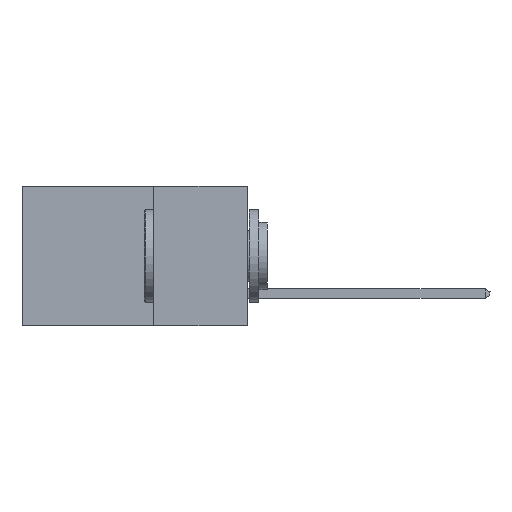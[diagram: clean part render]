
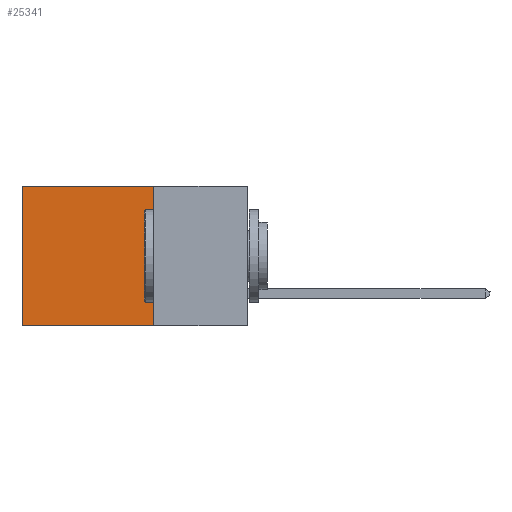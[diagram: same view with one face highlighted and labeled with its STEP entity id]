
A CAD part, left-side view. The second image highlights one B-rep face of the part: STEP entity #25341.
In plain terms, the highlighted planar face has unit normal (-1, 0, 0).
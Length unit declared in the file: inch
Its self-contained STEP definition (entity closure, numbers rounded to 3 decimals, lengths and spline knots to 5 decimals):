
#569 = LINE ( 'NONE', #8691, #19770 ) ;
#989 = EDGE_CURVE ( 'NONE', #20476, #14069, #7910, .T. ) ;
#1422 = VECTOR ( 'NONE', #15176, 39.37008 ) ;
#1435 = LINE ( 'NONE', #11559, #1422 ) ;
#1596 = AXIS2_PLACEMENT_3D ( 'NONE', #25720, #3160, #19194 ) ;
#2236 = VECTOR ( 'NONE', #13458, 39.37008 ) ;
#3160 = DIRECTION ( 'NONE',  ( 1., 0., 0. ) ) ;
#4863 = EDGE_CURVE ( 'NONE', #21299, #14069, #7465, .T. ) ;
#5056 = VERTEX_POINT ( 'NONE', #12913 ) ;
#5290 = PLANE ( 'NONE',  #1596 ) ;
#7465 = LINE ( 'NONE', #25747, #2236 ) ;
#7910 = LINE ( 'NONE', #13906, #25035 ) ;
#8293 = ORIENTED_EDGE ( 'NONE', *, *, #4863, .F. ) ;
#8383 = CARTESIAN_POINT ( 'NONE',  ( 0.2615, 0.6, -0.37 ) ) ;
#8691 = CARTESIAN_POINT ( 'NONE',  ( 0.2615, 0.25, -0.37 ) ) ;
#11559 = CARTESIAN_POINT ( 'NONE',  ( 0.2615, 0.25, 0. ) ) ;
#12913 = CARTESIAN_POINT ( 'NONE',  ( 0.2615, 0.25, 0. ) ) ;
#13458 = DIRECTION ( 'NONE',  ( 0., 1., 0. ) ) ;
#13906 = CARTESIAN_POINT ( 'NONE',  ( 0.2615, 0.6, -0.37 ) ) ;
#14069 = VERTEX_POINT ( 'NONE', #8383 ) ;
#15176 = DIRECTION ( 'NONE',  ( 0., 1., 0. ) ) ;
#16132 = CARTESIAN_POINT ( 'NONE',  ( 0.2615, 0.6, 0. ) ) ;
#16305 = CARTESIAN_POINT ( 'NONE',  ( 0.2615, 0.25, -0.37 ) ) ;
#17110 = DIRECTION ( 'NONE',  ( 0., 0., -1. ) ) ;
#17390 = ORIENTED_EDGE ( 'NONE', *, *, #989, .T. ) ;
#19194 = DIRECTION ( 'NONE',  ( 0., 0., -1. ) ) ;
#19270 = ORIENTED_EDGE ( 'NONE', *, *, #20813, .T. ) ;
#19770 = VECTOR ( 'NONE', #17110, 39.37008 ) ;
#20476 = VERTEX_POINT ( 'NONE', #16132 ) ;
#20813 = EDGE_CURVE ( 'NONE', #5056, #20476, #1435, .T. ) ;
#21299 = VERTEX_POINT ( 'NONE', #16305 ) ;
#21495 = EDGE_CURVE ( 'NONE', #5056, #21299, #569, .T. ) ;
#21979 = ORIENTED_EDGE ( 'NONE', *, *, #21495, .F. ) ;
#23473 = FACE_OUTER_BOUND ( 'NONE', #25352, .T. ) ;
#25035 = VECTOR ( 'NONE', #26339, 39.37008 ) ;
#25341 = ADVANCED_FACE ( 'NONE', ( #23473 ), #5290, .F. ) ;
#25352 = EDGE_LOOP ( 'NONE', ( #17390, #8293, #21979, #19270 ) ) ;
#25720 = CARTESIAN_POINT ( 'NONE',  ( 0.2615, 0.25, -0.37 ) ) ;
#25747 = CARTESIAN_POINT ( 'NONE',  ( 0.2615, 0.25, -0.37 ) ) ;
#26339 = DIRECTION ( 'NONE',  ( 0., 0., -1. ) ) ;
